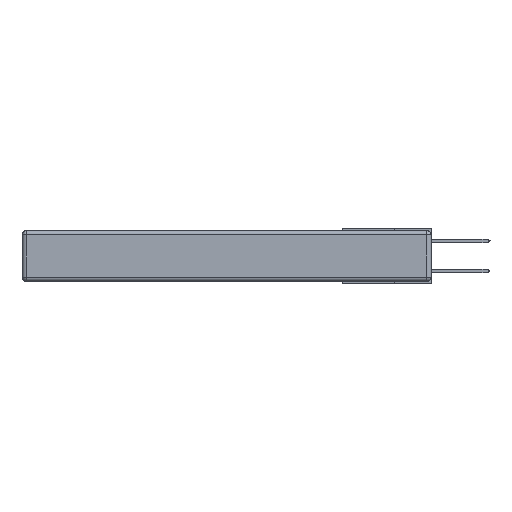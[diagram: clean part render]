
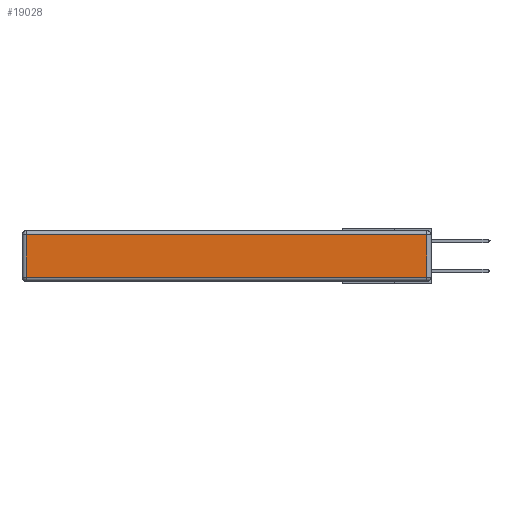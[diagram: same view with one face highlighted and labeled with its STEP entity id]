
A CAD part, left-side view. The second image highlights one B-rep face of the part: STEP entity #19028.
In plain terms, the highlighted planar face has unit normal (-1, 0, 0).
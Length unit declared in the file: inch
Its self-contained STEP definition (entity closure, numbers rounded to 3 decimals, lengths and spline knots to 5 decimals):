
#30 = CARTESIAN_POINT ( 'NONE',  ( 0., 2.72, -0.343 ) ) ;
#407 = CARTESIAN_POINT ( 'NONE',  ( 0., 0., -0.313 ) ) ;
#2280 = VECTOR ( 'NONE', #30568, 39.37008 ) ;
#2651 = EDGE_CURVE ( 'NONE', #15218, #12035, #18350, .T. ) ;
#2732 = CARTESIAN_POINT ( 'NONE',  ( 0., 0.03, -0.313 ) ) ;
#3124 = CARTESIAN_POINT ( 'NONE',  ( 0., 2.75, -0.03 ) ) ;
#4652 = ORIENTED_EDGE ( 'NONE', *, *, #22487, .T. ) ;
#5534 = DIRECTION ( 'NONE',  ( 0., 0., -1. ) ) ;
#11268 = FACE_OUTER_BOUND ( 'NONE', #30158, .T. ) ;
#11321 = ORIENTED_EDGE ( 'NONE', *, *, #14184, .T. ) ;
#12035 = VERTEX_POINT ( 'NONE', #2732 ) ;
#12820 = ORIENTED_EDGE ( 'NONE', *, *, #2651, .T. ) ;
#13335 = LINE ( 'NONE', #3124, #2280 ) ;
#14160 = LINE ( 'NONE', #30, #18000 ) ;
#14184 = EDGE_CURVE ( 'NONE', #15527, #15218, #14160, .T. ) ;
#14718 = LINE ( 'NONE', #24436, #19386 ) ;
#15218 = VERTEX_POINT ( 'NONE', #32357 ) ;
#15527 = VERTEX_POINT ( 'NONE', #18663 ) ;
#16931 = PLANE ( 'NONE',  #24360 ) ;
#18000 = VECTOR ( 'NONE', #5534, 39.37008 ) ;
#18350 = LINE ( 'NONE', #407, #21326 ) ;
#18663 = CARTESIAN_POINT ( 'NONE',  ( 0., 2.72, -0.03 ) ) ;
#19028 = ADVANCED_FACE ( 'NONE', ( #11268 ), #16931, .T. ) ;
#19386 = VECTOR ( 'NONE', #27534, 39.37008 ) ;
#19436 = DIRECTION ( 'NONE',  ( 0., -1., 0. ) ) ;
#19528 = CARTESIAN_POINT ( 'NONE',  ( 0., 0., -0.343 ) ) ;
#19747 = ORIENTED_EDGE ( 'NONE', *, *, #32056, .T. ) ;
#21326 = VECTOR ( 'NONE', #19436, 39.37008 ) ;
#22161 = VERTEX_POINT ( 'NONE', #22874 ) ;
#22487 = EDGE_CURVE ( 'NONE', #12035, #22161, #14718, .T. ) ;
#22640 = DIRECTION ( 'NONE',  ( 0., 0., 1. ) ) ;
#22874 = CARTESIAN_POINT ( 'NONE',  ( 0., 0.03, -0.03 ) ) ;
#24360 = AXIS2_PLACEMENT_3D ( 'NONE', #19528, #33196, #22640 ) ;
#24436 = CARTESIAN_POINT ( 'NONE',  ( 0., 0.03, -0.343 ) ) ;
#27534 = DIRECTION ( 'NONE',  ( 0., 0., 1. ) ) ;
#30158 = EDGE_LOOP ( 'NONE', ( #12820, #4652, #19747, #11321 ) ) ;
#30568 = DIRECTION ( 'NONE',  ( 0., 1., 0. ) ) ;
#32056 = EDGE_CURVE ( 'NONE', #22161, #15527, #13335, .T. ) ;
#32357 = CARTESIAN_POINT ( 'NONE',  ( 0., 2.72, -0.313 ) ) ;
#33196 = DIRECTION ( 'NONE',  ( -1., 0., 0. ) ) ;
